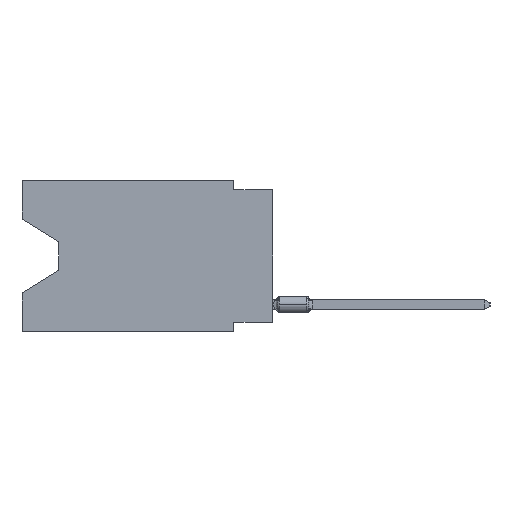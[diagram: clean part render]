
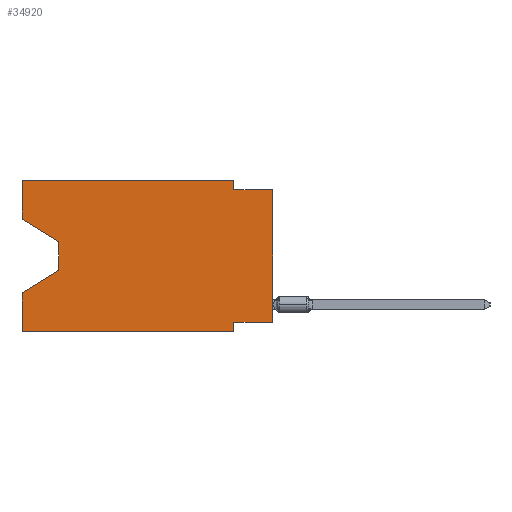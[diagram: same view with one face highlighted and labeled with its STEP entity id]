
A CAD part, left-side view. The second image highlights one B-rep face of the part: STEP entity #34920.
In plain terms, the highlighted planar face has unit normal (-1, 0, 0).
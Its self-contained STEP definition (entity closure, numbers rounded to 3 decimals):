
#137 = CARTESIAN_POINT ( 'NONE',  ( 0., 2.54, -9.906 ) ) ;
#474 = FACE_OUTER_BOUND ( 'NONE', #68764, .T. ) ;
#672 = DIRECTION ( 'NONE',  ( 0., 0.855, -0.519 ) ) ;
#3281 = DIRECTION ( 'NONE',  ( 0., 0., -1. ) ) ;
#4138 = VERTEX_POINT ( 'NONE', #54016 ) ;
#4828 = VECTOR ( 'NONE', #46568, 1000. ) ;
#6337 = CARTESIAN_POINT ( 'NONE',  ( 0., 13.97, -5.893 ) ) ;
#7425 = VERTEX_POINT ( 'NONE', #35785 ) ;
#8057 = ORIENTED_EDGE ( 'NONE', *, *, #74311, .T. ) ;
#8166 = ORIENTED_EDGE ( 'NONE', *, *, #45400, .F. ) ;
#8202 = VECTOR ( 'NONE', #56832, 1000. ) ;
#10104 = VECTOR ( 'NONE', #672, 1000. ) ;
#11830 = LINE ( 'NONE', #137, #46837 ) ;
#12338 = VERTEX_POINT ( 'NONE', #37732 ) ;
#12872 = EDGE_CURVE ( 'NONE', #55363, #43774, #28502, .T. ) ;
#13377 = LINE ( 'NONE', #59670, #42871 ) ;
#13384 = ORIENTED_EDGE ( 'NONE', *, *, #29377, .F. ) ;
#13740 = VECTOR ( 'NONE', #16696, 1000. ) ;
#15582 = VECTOR ( 'NONE', #64147, 1000. ) ;
#15766 = DIRECTION ( 'NONE',  ( 0., 1., 0. ) ) ;
#15888 = VERTEX_POINT ( 'NONE', #72220 ) ;
#16696 = DIRECTION ( 'NONE',  ( 0., 0., 1. ) ) ;
#17590 = CARTESIAN_POINT ( 'NONE',  ( 0., 16.383, 0. ) ) ;
#18130 = EDGE_CURVE ( 'NONE', #12338, #71323, #21953, .T. ) ;
#18314 = CARTESIAN_POINT ( 'NONE',  ( 0., 13.97, -4.013 ) ) ;
#18526 = DIRECTION ( 'NONE',  ( 1., 0., 0. ) ) ;
#20529 = LINE ( 'NONE', #72115, #33576 ) ;
#20841 = LINE ( 'NONE', #43829, #34106 ) ;
#21881 = VECTOR ( 'NONE', #71860, 1000. ) ;
#21953 = LINE ( 'NONE', #68258, #13740 ) ;
#22347 = EDGE_CURVE ( 'NONE', #59500, #7425, #58594, .T. ) ;
#23384 = ORIENTED_EDGE ( 'NONE', *, *, #29751, .F. ) ;
#26349 = EDGE_CURVE ( 'NONE', #4138, #31506, #11830, .T. ) ;
#26707 = ORIENTED_EDGE ( 'NONE', *, *, #41647, .T. ) ;
#27129 = ORIENTED_EDGE ( 'NONE', *, *, #12872, .F. ) ;
#27435 = LINE ( 'NONE', #50762, #68802 ) ;
#27702 = CARTESIAN_POINT ( 'NONE',  ( 0., 13.97, -4.013 ) ) ;
#28012 = EDGE_CURVE ( 'NONE', #36336, #15888, #73633, .T. ) ;
#28502 = LINE ( 'NONE', #34131, #4828 ) ;
#29076 = PLANE ( 'NONE',  #69362 ) ;
#29377 = EDGE_CURVE ( 'NONE', #12338, #4138, #27435, .T. ) ;
#29751 = EDGE_CURVE ( 'NONE', #43774, #36336, #20841, .T. ) ;
#31506 = VERTEX_POINT ( 'NONE', #68812 ) ;
#33349 = CARTESIAN_POINT ( 'NONE',  ( 0., 2.54, 0. ) ) ;
#33576 = VECTOR ( 'NONE', #43514, 1000. ) ;
#34106 = VECTOR ( 'NONE', #66781, 1000. ) ;
#34131 = CARTESIAN_POINT ( 'NONE',  ( 0., 16.383, 0. ) ) ;
#34920 = ADVANCED_FACE ( 'NONE', ( #474 ), #29076, .F. ) ;
#35785 = CARTESIAN_POINT ( 'NONE',  ( 0., 13.97, -5.893 ) ) ;
#36336 = VERTEX_POINT ( 'NONE', #71674 ) ;
#37314 = DIRECTION ( 'NONE',  ( 0., 0., -1. ) ) ;
#37732 = CARTESIAN_POINT ( 'NONE',  ( 0., 0., -9.271 ) ) ;
#37929 = CARTESIAN_POINT ( 'NONE',  ( 0., 16.383, -9.906 ) ) ;
#38802 = EDGE_CURVE ( 'NONE', #7425, #61987, #74084, .T. ) ;
#41040 = VECTOR ( 'NONE', #3281, 1000. ) ;
#41647 = EDGE_CURVE ( 'NONE', #63869, #31506, #13377, .T. ) ;
#42871 = VECTOR ( 'NONE', #65293, 1000. ) ;
#42895 = CARTESIAN_POINT ( 'NONE',  ( 0., 16.383, -2.546 ) ) ;
#43514 = DIRECTION ( 'NONE',  ( 0., -1., 0. ) ) ;
#43770 = ORIENTED_EDGE ( 'NONE', *, *, #38802, .T. ) ;
#43774 = VERTEX_POINT ( 'NONE', #17590 ) ;
#43829 = CARTESIAN_POINT ( 'NONE',  ( 0., 16.383, 0. ) ) ;
#45053 = EDGE_CURVE ( 'NONE', #15888, #71323, #20529, .T. ) ;
#45400 = EDGE_CURVE ( 'NONE', #63869, #61987, #46859, .T. ) ;
#46105 = CARTESIAN_POINT ( 'NONE',  ( 0., 16.383, 0. ) ) ;
#46448 = DIRECTION ( 'NONE',  ( 0., 0., -1. ) ) ;
#46568 = DIRECTION ( 'NONE',  ( 0., 0., 1. ) ) ;
#46837 = VECTOR ( 'NONE', #46448, 1000. ) ;
#46859 = LINE ( 'NONE', #46105, #15582 ) ;
#50762 = CARTESIAN_POINT ( 'NONE',  ( 0., 0., -9.271 ) ) ;
#54016 = CARTESIAN_POINT ( 'NONE',  ( 0., 2.54, -9.271 ) ) ;
#55363 = VERTEX_POINT ( 'NONE', #70037 ) ;
#56635 = ORIENTED_EDGE ( 'NONE', *, *, #28012, .F. ) ;
#56832 = DIRECTION ( 'NONE',  ( 0., 0., -1. ) ) ;
#57289 = CARTESIAN_POINT ( 'NONE',  ( 0., 16.383, -7.36 ) ) ;
#58594 = LINE ( 'NONE', #18314, #8202 ) ;
#59500 = VERTEX_POINT ( 'NONE', #27702 ) ;
#59670 = CARTESIAN_POINT ( 'NONE',  ( 0., 16.383, -9.906 ) ) ;
#60457 = CARTESIAN_POINT ( 'NONE',  ( 0., 0., -0.635 ) ) ;
#61436 = ORIENTED_EDGE ( 'NONE', *, *, #22347, .T. ) ;
#61987 = VERTEX_POINT ( 'NONE', #57289 ) ;
#62552 = ORIENTED_EDGE ( 'NONE', *, *, #45053, .F. ) ;
#63869 = VERTEX_POINT ( 'NONE', #37929 ) ;
#64147 = DIRECTION ( 'NONE',  ( 0., 0., 1. ) ) ;
#65293 = DIRECTION ( 'NONE',  ( 0., -1., 0. ) ) ;
#66781 = DIRECTION ( 'NONE',  ( 0., -1., 0. ) ) ;
#66890 = ORIENTED_EDGE ( 'NONE', *, *, #18130, .T. ) ;
#67867 = ORIENTED_EDGE ( 'NONE', *, *, #26349, .F. ) ;
#68258 = CARTESIAN_POINT ( 'NONE',  ( 0., 0., 0. ) ) ;
#68764 = EDGE_LOOP ( 'NONE', ( #8057, #61436, #43770, #8166, #26707, #67867, #13384, #66890, #62552, #56635, #23384, #27129 ) ) ;
#68802 = VECTOR ( 'NONE', #15766, 1000. ) ;
#68812 = CARTESIAN_POINT ( 'NONE',  ( 0., 2.54, -9.906 ) ) ;
#69362 = AXIS2_PLACEMENT_3D ( 'NONE', #70085, #18526, #37314 ) ;
#70037 = CARTESIAN_POINT ( 'NONE',  ( 0., 16.383, -2.546 ) ) ;
#70085 = CARTESIAN_POINT ( 'NONE',  ( 0., 16.383, 0. ) ) ;
#71323 = VERTEX_POINT ( 'NONE', #60457 ) ;
#71479 = LINE ( 'NONE', #42895, #21881 ) ;
#71674 = CARTESIAN_POINT ( 'NONE',  ( 0., 2.54, 0. ) ) ;
#71860 = DIRECTION ( 'NONE',  ( 0., -0.855, -0.519 ) ) ;
#72115 = CARTESIAN_POINT ( 'NONE',  ( 0., 0., -0.635 ) ) ;
#72220 = CARTESIAN_POINT ( 'NONE',  ( 0., 2.54, -0.635 ) ) ;
#73633 = LINE ( 'NONE', #33349, #41040 ) ;
#74084 = LINE ( 'NONE', #6337, #10104 ) ;
#74311 = EDGE_CURVE ( 'NONE', #55363, #59500, #71479, .T. ) ;
